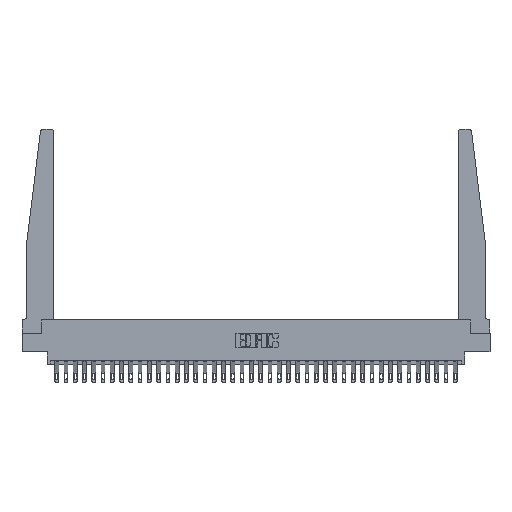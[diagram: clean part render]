
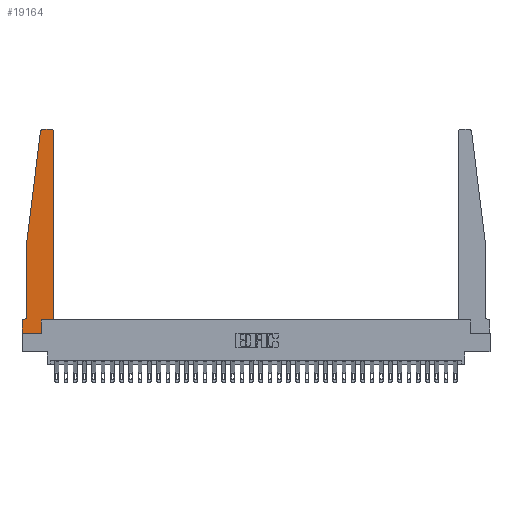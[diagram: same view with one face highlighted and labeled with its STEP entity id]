
A CAD part, top view. The second image highlights one B-rep face of the part: STEP entity #19164.
In plain terms, the highlighted planar face has unit normal (0, 0, 1).
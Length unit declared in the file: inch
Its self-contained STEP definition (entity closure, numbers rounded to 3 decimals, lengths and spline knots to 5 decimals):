
#49 = VERTEX_POINT ( 'NONE', #33416 ) ;
#691 = ORIENTED_EDGE ( 'NONE', *, *, #1130, .T. ) ;
#1130 = EDGE_CURVE ( 'NONE', #22354, #21286, #32180, .T. ) ;
#1319 = DIRECTION ( 'NONE',  ( 1., 0., 0. ) ) ;
#1714 = CARTESIAN_POINT ( 'NONE',  ( 0.065, 0.1875, 0.37 ) ) ;
#2239 = VECTOR ( 'NONE', #19468, 39.37008 ) ;
#2691 = ORIENTED_EDGE ( 'NONE', *, *, #19008, .T. ) ;
#2729 = AXIS2_PLACEMENT_3D ( 'NONE', #13736, #31942, #16369 ) ;
#3812 = EDGE_CURVE ( 'NONE', #11876, #32397, #25539, .T. ) ;
#4285 = ORIENTED_EDGE ( 'NONE', *, *, #21610, .T. ) ;
#4733 = VECTOR ( 'NONE', #20495, 39.37008 ) ;
#5812 = CARTESIAN_POINT ( 'NONE',  ( 0.395, 2.72, 0.37 ) ) ;
#5997 = VERTEX_POINT ( 'NONE', #26518 ) ;
#6419 = LINE ( 'NONE', #10054, #11699 ) ;
#6996 = VERTEX_POINT ( 'NONE', #28897 ) ;
#7098 = CARTESIAN_POINT ( 'NONE',  ( 0.425, 0.18, 0.37 ) ) ;
#7170 = CIRCLE ( 'NONE', #14624, 0.03 ) ;
#7487 = CARTESIAN_POINT ( 'NONE',  ( 0.065, 1.25, 0.37 ) ) ;
#7505 = CARTESIAN_POINT ( 'NONE',  ( 0.425, 0.18, 0.37 ) ) ;
#7620 = ORIENTED_EDGE ( 'NONE', *, *, #21818, .T. ) ;
#7732 = CARTESIAN_POINT ( 'NONE',  ( 0.27653, 2.72, 0.37 ) ) ;
#7923 = EDGE_CURVE ( 'NONE', #11763, #11876, #27974, .T. ) ;
#8387 = LINE ( 'NONE', #1714, #29152 ) ;
#8444 = DIRECTION ( 'NONE',  ( 1., 0., 0. ) ) ;
#8541 = VECTOR ( 'NONE', #32705, 39.37008 ) ;
#9152 = LINE ( 'NONE', #16845, #2239 ) ;
#9349 = LINE ( 'NONE', #30105, #8541 ) ;
#9801 = DIRECTION ( 'NONE',  ( 0., -1., 0. ) ) ;
#9867 = EDGE_CURVE ( 'NONE', #5997, #6996, #28301, .T. ) ;
#9964 = CARTESIAN_POINT ( 'NONE',  ( 0.425, 0.18, 0.37 ) ) ;
#10054 = CARTESIAN_POINT ( 'NONE',  ( 0., 0., 0.37 ) ) ;
#10349 = DIRECTION ( 'NONE',  ( 1., 0., 0. ) ) ;
#10939 = CARTESIAN_POINT ( 'NONE',  ( 0.065, 0.2375, 0.37 ) ) ;
#11567 = PLANE ( 'NONE',  #21948 ) ;
#11699 = VECTOR ( 'NONE', #30872, 39.37008 ) ;
#11763 = VERTEX_POINT ( 'NONE', #14610 ) ;
#11779 = LINE ( 'NONE', #17068, #18721 ) ;
#11876 = VERTEX_POINT ( 'NONE', #9964 ) ;
#11957 = EDGE_LOOP ( 'NONE', ( #31997, #7620, #15400, #691, #2691, #4285, #19707, #27777, #12192, #15014, #13458, #13109 ) ) ;
#12192 = ORIENTED_EDGE ( 'NONE', *, *, #12855, .T. ) ;
#12342 = CARTESIAN_POINT ( 'NONE',  ( 0.25, 2.75, 0.37 ) ) ;
#12855 = EDGE_CURVE ( 'NONE', #26310, #11763, #11779, .T. ) ;
#13109 = ORIENTED_EDGE ( 'NONE', *, *, #14429, .T. ) ;
#13336 = CARTESIAN_POINT ( 'NONE',  ( 0.2605, 0., 0.37 ) ) ;
#13458 = ORIENTED_EDGE ( 'NONE', *, *, #3812, .T. ) ;
#13657 = VERTEX_POINT ( 'NONE', #30784 ) ;
#13736 = CARTESIAN_POINT ( 'NONE',  ( 0.015, 0.2375, 0.37 ) ) ;
#14429 = EDGE_CURVE ( 'NONE', #32397, #5997, #7170, .T. ) ;
#14610 = CARTESIAN_POINT ( 'NONE',  ( 0.2605, 0.18, 0.37 ) ) ;
#14624 = AXIS2_PLACEMENT_3D ( 'NONE', #5812, #24054, #8444 ) ;
#15014 = ORIENTED_EDGE ( 'NONE', *, *, #7923, .T. ) ;
#15392 = VERTEX_POINT ( 'NONE', #17421 ) ;
#15400 = ORIENTED_EDGE ( 'NONE', *, *, #22065, .T. ) ;
#15639 = CARTESIAN_POINT ( 'NONE',  ( 0.015, 0.1875, 0.37 ) ) ;
#16369 = DIRECTION ( 'NONE',  ( -1., 0., 0. ) ) ;
#16505 = CIRCLE ( 'NONE', #29608, 0.03 ) ;
#16845 = CARTESIAN_POINT ( 'NONE',  ( 0.065, 1.25, 0.37 ) ) ;
#16935 = DIRECTION ( 'NONE',  ( 0., 0., 1. ) ) ;
#17068 = CARTESIAN_POINT ( 'NONE',  ( 0.2605, 0.18, 0.37 ) ) ;
#17421 = CARTESIAN_POINT ( 'NONE',  ( 0., 0.1875, 0.37 ) ) ;
#17591 = DIRECTION ( 'NONE',  ( -1., 0., 0. ) ) ;
#17915 = EDGE_CURVE ( 'NONE', #49, #26310, #9349, .T. ) ;
#18721 = VECTOR ( 'NONE', #19697, 39.37008 ) ;
#19008 = EDGE_CURVE ( 'NONE', #21286, #29844, #32067, .T. ) ;
#19164 = ADVANCED_FACE ( 'NONE', ( #28027 ), #11567, .T. ) ;
#19468 = DIRECTION ( 'NONE',  ( -0.122, -0.992, 0. ) ) ;
#19697 = DIRECTION ( 'NONE',  ( 0., 1., 0. ) ) ;
#19707 = ORIENTED_EDGE ( 'NONE', *, *, #19960, .T. ) ;
#19960 = EDGE_CURVE ( 'NONE', #15392, #49, #6419, .T. ) ;
#20452 = CARTESIAN_POINT ( 'NONE',  ( 0.425, 2.72, 0.37 ) ) ;
#20495 = DIRECTION ( 'NONE',  ( 0., 1., 0. ) ) ;
#21286 = VERTEX_POINT ( 'NONE', #10939 ) ;
#21401 = VECTOR ( 'NONE', #17591, 39.37008 ) ;
#21610 = EDGE_CURVE ( 'NONE', #29844, #15392, #8387, .T. ) ;
#21818 = EDGE_CURVE ( 'NONE', #6996, #13657, #16505, .T. ) ;
#21948 = AXIS2_PLACEMENT_3D ( 'NONE', #32507, #16935, #1319 ) ;
#22065 = EDGE_CURVE ( 'NONE', #13657, #22354, #9152, .T. ) ;
#22354 = VERTEX_POINT ( 'NONE', #7487 ) ;
#24054 = DIRECTION ( 'NONE',  ( 0., 0., 1. ) ) ;
#25294 = VECTOR ( 'NONE', #9801, 39.37008 ) ;
#25539 = LINE ( 'NONE', #7505, #4733 ) ;
#25975 = DIRECTION ( 'NONE',  ( 0., 0., 1. ) ) ;
#26310 = VERTEX_POINT ( 'NONE', #13336 ) ;
#26518 = CARTESIAN_POINT ( 'NONE',  ( 0.395, 2.75, 0.37 ) ) ;
#27179 = VECTOR ( 'NONE', #27941, 39.37008 ) ;
#27777 = ORIENTED_EDGE ( 'NONE', *, *, #17915, .T. ) ;
#27941 = DIRECTION ( 'NONE',  ( 1., 0., 0. ) ) ;
#27974 = LINE ( 'NONE', #7098, #27179 ) ;
#28027 = FACE_OUTER_BOUND ( 'NONE', #11957, .T. ) ;
#28301 = LINE ( 'NONE', #12342, #21401 ) ;
#28897 = CARTESIAN_POINT ( 'NONE',  ( 0.27653, 2.75, 0.37 ) ) ;
#29152 = VECTOR ( 'NONE', #32879, 39.37008 ) ;
#29608 = AXIS2_PLACEMENT_3D ( 'NONE', #7732, #25975, #10349 ) ;
#29844 = VERTEX_POINT ( 'NONE', #15639 ) ;
#30105 = CARTESIAN_POINT ( 'NONE',  ( 0., 0., 0.37 ) ) ;
#30784 = CARTESIAN_POINT ( 'NONE',  ( 0.24675, 2.72367, 0.37 ) ) ;
#30872 = DIRECTION ( 'NONE',  ( 0., -1., 0. ) ) ;
#31942 = DIRECTION ( 'NONE',  ( 0., 0., -1. ) ) ;
#31997 = ORIENTED_EDGE ( 'NONE', *, *, #9867, .T. ) ;
#32067 = CIRCLE ( 'NONE', #2729, 0.05 ) ;
#32180 = LINE ( 'NONE', #33121, #25294 ) ;
#32397 = VERTEX_POINT ( 'NONE', #20452 ) ;
#32507 = CARTESIAN_POINT ( 'NONE',  ( 0., 0.1875, 0.37 ) ) ;
#32705 = DIRECTION ( 'NONE',  ( 1., 0., 0. ) ) ;
#32879 = DIRECTION ( 'NONE',  ( -1., 0., 0. ) ) ;
#33121 = CARTESIAN_POINT ( 'NONE',  ( 0.065, 1.25, 0.37 ) ) ;
#33416 = CARTESIAN_POINT ( 'NONE',  ( 0., 0., 0.37 ) ) ;
